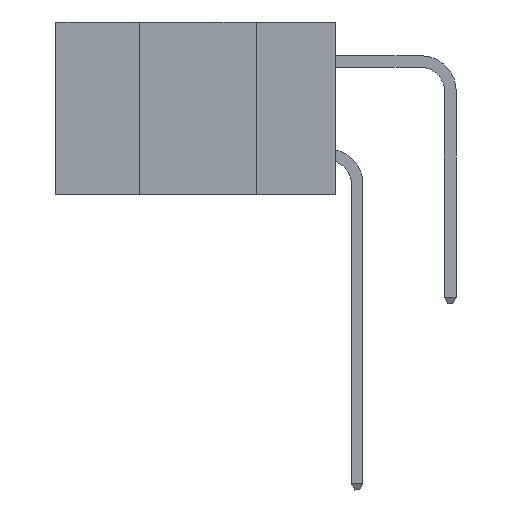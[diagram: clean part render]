
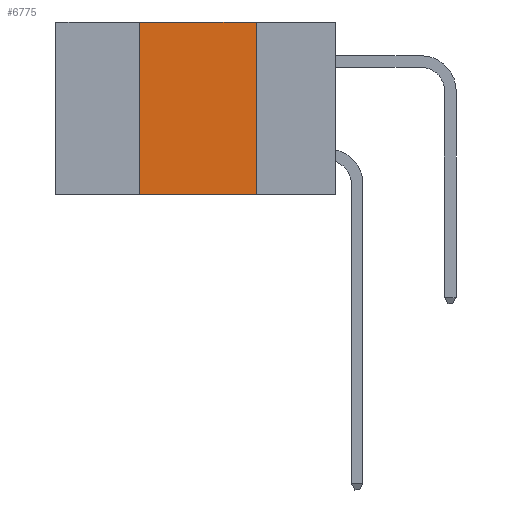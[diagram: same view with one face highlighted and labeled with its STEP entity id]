
A CAD part, left-side view. The second image highlights one B-rep face of the part: STEP entity #6775.
In plain terms, the highlighted planar face has unit normal (-1, 0, 0).
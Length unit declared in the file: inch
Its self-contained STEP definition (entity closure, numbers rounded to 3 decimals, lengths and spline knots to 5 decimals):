
#165 = DIRECTION ( 'NONE',  ( 0., -1., 0. ) ) ;
#1178 = VERTEX_POINT ( 'NONE', #11598 ) ;
#1351 = VECTOR ( 'NONE', #8183, 39.37008 ) ;
#2692 = CARTESIAN_POINT ( 'NONE',  ( 0., 0.6, 0. ) ) ;
#2758 = PLANE ( 'NONE',  #16221 ) ;
#4297 = EDGE_CURVE ( 'NONE', #1178, #16276, #13794, .T. ) ;
#4387 = DIRECTION ( 'NONE',  ( 0., 0., -1. ) ) ;
#4624 = CARTESIAN_POINT ( 'NONE',  ( 0., 0.6, -0.37 ) ) ;
#4687 = EDGE_LOOP ( 'NONE', ( #7718, #8568, #7732, #8027 ) ) ;
#5108 = LINE ( 'NONE', #15658, #1351 ) ;
#6775 = ADVANCED_FACE ( 'NONE', ( #12512 ), #2758, .F. ) ;
#7718 = ORIENTED_EDGE ( 'NONE', *, *, #17480, .F. ) ;
#7732 = ORIENTED_EDGE ( 'NONE', *, *, #13698, .F. ) ;
#7735 = VERTEX_POINT ( 'NONE', #16410 ) ;
#8027 = ORIENTED_EDGE ( 'NONE', *, *, #4297, .T. ) ;
#8183 = DIRECTION ( 'NONE',  ( 0., 0., 1. ) ) ;
#8568 = ORIENTED_EDGE ( 'NONE', *, *, #11963, .F. ) ;
#8831 = VECTOR ( 'NONE', #16694, 39.37008 ) ;
#8890 = CARTESIAN_POINT ( 'NONE',  ( 0., 0.17, 0. ) ) ;
#10356 = VECTOR ( 'NONE', #165, 39.37008 ) ;
#11412 = VECTOR ( 'NONE', #16380, 39.37008 ) ;
#11598 = CARTESIAN_POINT ( 'NONE',  ( 0., 0.42, -0.37 ) ) ;
#11896 = VERTEX_POINT ( 'NONE', #18346 ) ;
#11963 = EDGE_CURVE ( 'NONE', #11896, #7735, #12989, .T. ) ;
#12512 = FACE_OUTER_BOUND ( 'NONE', #4687, .T. ) ;
#12989 = LINE ( 'NONE', #17006, #10356 ) ;
#13491 = DIRECTION ( 'NONE',  ( 1., 0., 0. ) ) ;
#13698 = EDGE_CURVE ( 'NONE', #1178, #11896, #5108, .T. ) ;
#13794 = LINE ( 'NONE', #4624, #8831 ) ;
#15377 = LINE ( 'NONE', #8890, #11412 ) ;
#15658 = CARTESIAN_POINT ( 'NONE',  ( 0., 0.42, 0. ) ) ;
#16221 = AXIS2_PLACEMENT_3D ( 'NONE', #2692, #13491, #4387 ) ;
#16276 = VERTEX_POINT ( 'NONE', #19700 ) ;
#16380 = DIRECTION ( 'NONE',  ( 0., 0., -1. ) ) ;
#16410 = CARTESIAN_POINT ( 'NONE',  ( 0., 0.17, 0. ) ) ;
#16694 = DIRECTION ( 'NONE',  ( 0., -1., 0. ) ) ;
#17006 = CARTESIAN_POINT ( 'NONE',  ( 0., 0.6, 0. ) ) ;
#17480 = EDGE_CURVE ( 'NONE', #7735, #16276, #15377, .T. ) ;
#18346 = CARTESIAN_POINT ( 'NONE',  ( 0., 0.42, 0. ) ) ;
#19700 = CARTESIAN_POINT ( 'NONE',  ( 0., 0.17, -0.37 ) ) ;
